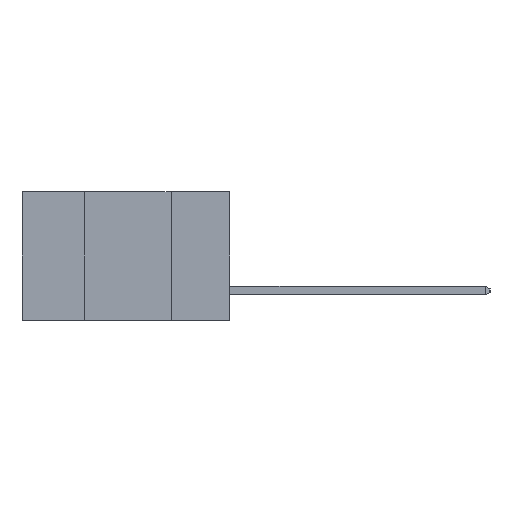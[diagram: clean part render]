
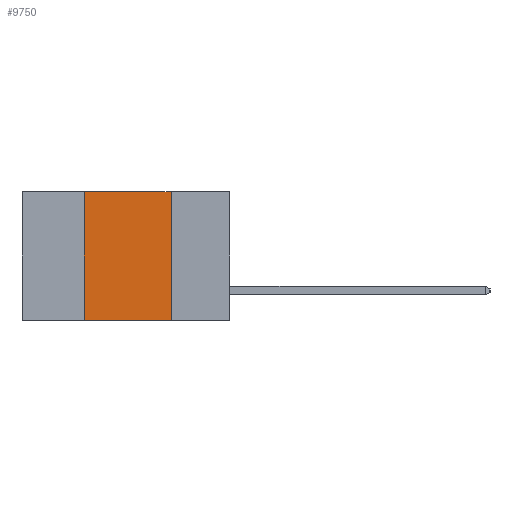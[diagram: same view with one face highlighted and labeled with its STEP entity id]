
A CAD part, left-side view. The second image highlights one B-rep face of the part: STEP entity #9750.
In plain terms, the highlighted planar face has unit normal (-1, 0, 0).
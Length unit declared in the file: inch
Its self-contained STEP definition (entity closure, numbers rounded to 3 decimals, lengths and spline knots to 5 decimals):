
#1076 = AXIS2_PLACEMENT_3D ( 'NONE', #3198, #11336, #6017 ) ;
#1434 = VERTEX_POINT ( 'NONE', #6887 ) ;
#1651 = ORIENTED_EDGE ( 'NONE', *, *, #4619, .F. ) ;
#1764 = EDGE_CURVE ( 'NONE', #7522, #1434, #8980, .T. ) ;
#1881 = LINE ( 'NONE', #4458, #11835 ) ;
#2184 = ORIENTED_EDGE ( 'NONE', *, *, #1764, .F. ) ;
#3198 = CARTESIAN_POINT ( 'NONE',  ( 0., 0.6, 0. ) ) ;
#3994 = EDGE_CURVE ( 'NONE', #9850, #1434, #6440, .T. ) ;
#4157 = VECTOR ( 'NONE', #11195, 39.37008 ) ;
#4451 = CARTESIAN_POINT ( 'NONE',  ( 0., 0.42, -0.37 ) ) ;
#4458 = CARTESIAN_POINT ( 'NONE',  ( 0., 0.6, 0. ) ) ;
#4505 = CARTESIAN_POINT ( 'NONE',  ( 0., 0.6, -0.37 ) ) ;
#4619 = EDGE_CURVE ( 'NONE', #9850, #7635, #8921, .T. ) ;
#5087 = PLANE ( 'NONE',  #1076 ) ;
#5628 = ORIENTED_EDGE ( 'NONE', *, *, #7560, .F. ) ;
#5940 = FACE_OUTER_BOUND ( 'NONE', #7986, .T. ) ;
#6017 = DIRECTION ( 'NONE',  ( 0., 0., -1. ) ) ;
#6440 = LINE ( 'NONE', #4505, #10876 ) ;
#6885 = ORIENTED_EDGE ( 'NONE', *, *, #3994, .T. ) ;
#6887 = CARTESIAN_POINT ( 'NONE',  ( 0., 0.17, -0.37 ) ) ;
#7011 = CARTESIAN_POINT ( 'NONE',  ( 0., 0.42, -0.37 ) ) ;
#7501 = CARTESIAN_POINT ( 'NONE',  ( 0., 0.17, -0.37 ) ) ;
#7522 = VERTEX_POINT ( 'NONE', #11579 ) ;
#7560 = EDGE_CURVE ( 'NONE', #7635, #7522, #1881, .T. ) ;
#7635 = VERTEX_POINT ( 'NONE', #10817 ) ;
#7986 = EDGE_LOOP ( 'NONE', ( #2184, #5628, #1651, #6885 ) ) ;
#8107 = DIRECTION ( 'NONE',  ( 0., 0., 1. ) ) ;
#8921 = LINE ( 'NONE', #4451, #9198 ) ;
#8980 = LINE ( 'NONE', #7501, #4157 ) ;
#9198 = VECTOR ( 'NONE', #8107, 39.37008 ) ;
#9750 = ADVANCED_FACE ( 'NONE', ( #5940 ), #5087, .F. ) ;
#9850 = VERTEX_POINT ( 'NONE', #7011 ) ;
#9854 = DIRECTION ( 'NONE',  ( 0., -1., 0. ) ) ;
#9893 = DIRECTION ( 'NONE',  ( 0., -1., 0. ) ) ;
#10817 = CARTESIAN_POINT ( 'NONE',  ( 0., 0.42, 0. ) ) ;
#10876 = VECTOR ( 'NONE', #9893, 39.37008 ) ;
#11195 = DIRECTION ( 'NONE',  ( 0., 0., -1. ) ) ;
#11336 = DIRECTION ( 'NONE',  ( 1., 0., 0. ) ) ;
#11579 = CARTESIAN_POINT ( 'NONE',  ( 0., 0.17, 0. ) ) ;
#11835 = VECTOR ( 'NONE', #9854, 39.37008 ) ;
